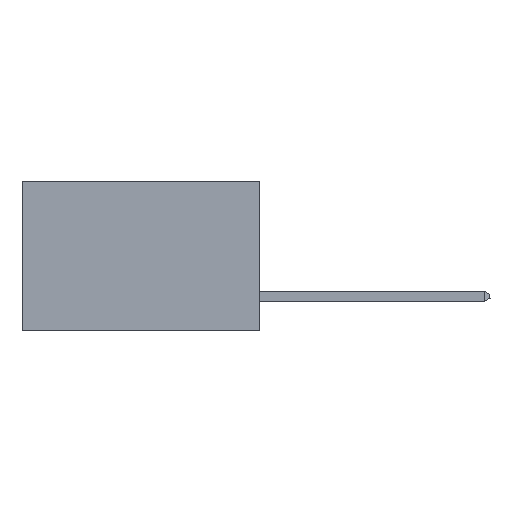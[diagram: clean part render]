
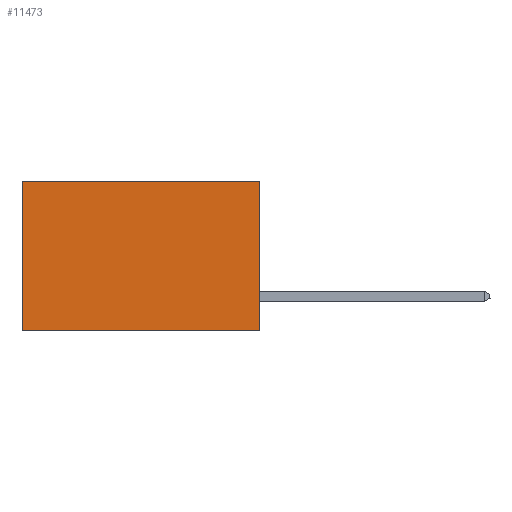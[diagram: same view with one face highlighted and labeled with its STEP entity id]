
A CAD part, left-side view. The second image highlights one B-rep face of the part: STEP entity #11473.
In plain terms, the highlighted planar face has unit normal (-1, 0, 0).
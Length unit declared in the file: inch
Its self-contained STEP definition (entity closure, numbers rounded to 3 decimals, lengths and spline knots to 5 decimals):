
#1029 = VECTOR ( 'NONE', #11419, 39.37008 ) ;
#1622 = CARTESIAN_POINT ( 'NONE',  ( 0.277, 0.59, -0.37 ) ) ;
#1659 = FACE_OUTER_BOUND ( 'NONE', #12900, .T. ) ;
#1695 = ORIENTED_EDGE ( 'NONE', *, *, #7351, .F. ) ;
#2285 = EDGE_CURVE ( 'NONE', #14664, #7643, #13419, .T. ) ;
#2696 = CARTESIAN_POINT ( 'NONE',  ( 0.277, 0., -0.37 ) ) ;
#3089 = CARTESIAN_POINT ( 'NONE',  ( 0.277, 0.59, 0. ) ) ;
#3552 = VECTOR ( 'NONE', #6250, 39.37008 ) ;
#4045 = VECTOR ( 'NONE', #11746, 39.37008 ) ;
#4054 = CARTESIAN_POINT ( 'NONE',  ( 0.277, 0., -0.37 ) ) ;
#4074 = DIRECTION ( 'NONE',  ( 0., 0., -1. ) ) ;
#4281 = CARTESIAN_POINT ( 'NONE',  ( 0.277, 0., -0.37 ) ) ;
#4634 = CARTESIAN_POINT ( 'NONE',  ( 0.277, 0., 0. ) ) ;
#5600 = DIRECTION ( 'NONE',  ( 0., 0., -1. ) ) ;
#6133 = LINE ( 'NONE', #4054, #12544 ) ;
#6250 = DIRECTION ( 'NONE',  ( 0., 0., -1. ) ) ;
#6465 = AXIS2_PLACEMENT_3D ( 'NONE', #4281, #13274, #5600 ) ;
#7303 = VERTEX_POINT ( 'NONE', #4634 ) ;
#7351 = EDGE_CURVE ( 'NONE', #7303, #13221, #6133, .T. ) ;
#7643 = VERTEX_POINT ( 'NONE', #1622 ) ;
#7969 = LINE ( 'NONE', #10108, #1029 ) ;
#9022 = ORIENTED_EDGE ( 'NONE', *, *, #14290, .T. ) ;
#10108 = CARTESIAN_POINT ( 'NONE',  ( 0.277, 0., 0. ) ) ;
#10497 = ORIENTED_EDGE ( 'NONE', *, *, #2285, .T. ) ;
#11419 = DIRECTION ( 'NONE',  ( 0., 1., 0. ) ) ;
#11473 = ADVANCED_FACE ( 'NONE', ( #1659 ), #11978, .F. ) ;
#11746 = DIRECTION ( 'NONE',  ( 0., 1., 0. ) ) ;
#11767 = CARTESIAN_POINT ( 'NONE',  ( 0.277, 0., -0.37 ) ) ;
#11978 = PLANE ( 'NONE',  #6465 ) ;
#12544 = VECTOR ( 'NONE', #4074, 39.37008 ) ;
#12900 = EDGE_LOOP ( 'NONE', ( #10497, #16242, #1695, #9022 ) ) ;
#13221 = VERTEX_POINT ( 'NONE', #11767 ) ;
#13274 = DIRECTION ( 'NONE',  ( 1., 0., 0. ) ) ;
#13419 = LINE ( 'NONE', #13969, #3552 ) ;
#13868 = LINE ( 'NONE', #2696, #4045 ) ;
#13969 = CARTESIAN_POINT ( 'NONE',  ( 0.277, 0.59, -0.37 ) ) ;
#14290 = EDGE_CURVE ( 'NONE', #7303, #14664, #7969, .T. ) ;
#14664 = VERTEX_POINT ( 'NONE', #3089 ) ;
#16242 = ORIENTED_EDGE ( 'NONE', *, *, #16406, .F. ) ;
#16406 = EDGE_CURVE ( 'NONE', #13221, #7643, #13868, .T. ) ;
